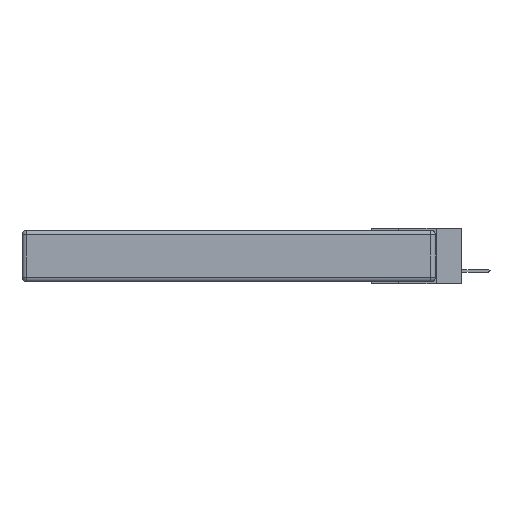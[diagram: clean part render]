
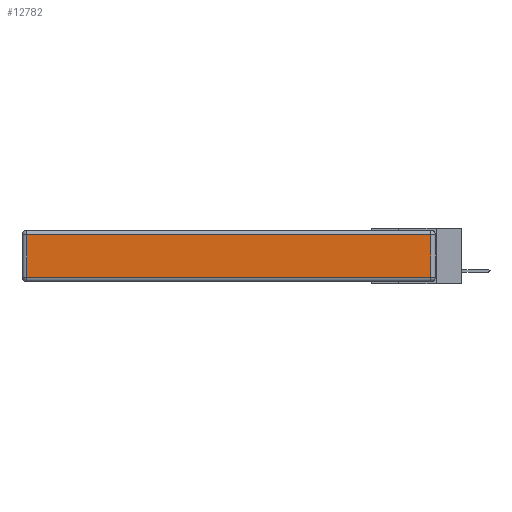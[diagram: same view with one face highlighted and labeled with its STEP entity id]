
A CAD part, left-side view. The second image highlights one B-rep face of the part: STEP entity #12782.
In plain terms, the highlighted planar face has unit normal (-1, 0, 0).
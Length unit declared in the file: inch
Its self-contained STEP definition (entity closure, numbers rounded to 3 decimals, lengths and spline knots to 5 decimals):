
#354 = AXIS2_PLACEMENT_3D ( 'NONE', #14810, #17245, #8255 ) ;
#1085 = PLANE ( 'NONE',  #354 ) ;
#1096 = LINE ( 'NONE', #9622, #18818 ) ;
#1106 = ORIENTED_EDGE ( 'NONE', *, *, #4860, .T. ) ;
#2792 = LINE ( 'NONE', #19148, #17256 ) ;
#4349 = VERTEX_POINT ( 'NONE', #11394 ) ;
#4860 = EDGE_CURVE ( 'NONE', #15060, #25251, #29315, .T. ) ;
#5765 = EDGE_CURVE ( 'NONE', #25251, #4349, #1096, .T. ) ;
#6040 = CARTESIAN_POINT ( 'NONE',  ( 0., 0.03, -0.343 ) ) ;
#8215 = CARTESIAN_POINT ( 'NONE',  ( 0., 0.03, -0.313 ) ) ;
#8255 = DIRECTION ( 'NONE',  ( 0., 0., 1. ) ) ;
#9214 = ORIENTED_EDGE ( 'NONE', *, *, #9876, .T. ) ;
#9622 = CARTESIAN_POINT ( 'NONE',  ( 0., 2.75, -0.03 ) ) ;
#9876 = EDGE_CURVE ( 'NONE', #25744, #15060, #14842, .T. ) ;
#10299 = EDGE_LOOP ( 'NONE', ( #9214, #1106, #17531, #15236 ) ) ;
#10909 = DIRECTION ( 'NONE',  ( 0., -1., 0. ) ) ;
#11394 = CARTESIAN_POINT ( 'NONE',  ( 0., 2.72, -0.03 ) ) ;
#12100 = CARTESIAN_POINT ( 'NONE',  ( 0., 2.72, -0.313 ) ) ;
#12782 = ADVANCED_FACE ( 'NONE', ( #26210 ), #1085, .T. ) ;
#14171 = CARTESIAN_POINT ( 'NONE',  ( 0., 0.03, -0.03 ) ) ;
#14810 = CARTESIAN_POINT ( 'NONE',  ( 0., 0., -0.343 ) ) ;
#14842 = LINE ( 'NONE', #24827, #18092 ) ;
#15060 = VERTEX_POINT ( 'NONE', #8215 ) ;
#15236 = ORIENTED_EDGE ( 'NONE', *, *, #17804, .T. ) ;
#16694 = DIRECTION ( 'NONE',  ( 0., 0., -1. ) ) ;
#17245 = DIRECTION ( 'NONE',  ( -1., 0., 0. ) ) ;
#17256 = VECTOR ( 'NONE', #16694, 39.37008 ) ;
#17531 = ORIENTED_EDGE ( 'NONE', *, *, #5765, .T. ) ;
#17804 = EDGE_CURVE ( 'NONE', #4349, #25744, #2792, .T. ) ;
#18092 = VECTOR ( 'NONE', #10909, 39.37008 ) ;
#18818 = VECTOR ( 'NONE', #23664, 39.37008 ) ;
#19148 = CARTESIAN_POINT ( 'NONE',  ( 0., 2.72, -0.343 ) ) ;
#22593 = DIRECTION ( 'NONE',  ( 0., 0., 1. ) ) ;
#23664 = DIRECTION ( 'NONE',  ( 0., 1., 0. ) ) ;
#24566 = VECTOR ( 'NONE', #22593, 39.37008 ) ;
#24827 = CARTESIAN_POINT ( 'NONE',  ( 0., 0., -0.313 ) ) ;
#25251 = VERTEX_POINT ( 'NONE', #14171 ) ;
#25744 = VERTEX_POINT ( 'NONE', #12100 ) ;
#26210 = FACE_OUTER_BOUND ( 'NONE', #10299, .T. ) ;
#29315 = LINE ( 'NONE', #6040, #24566 ) ;
